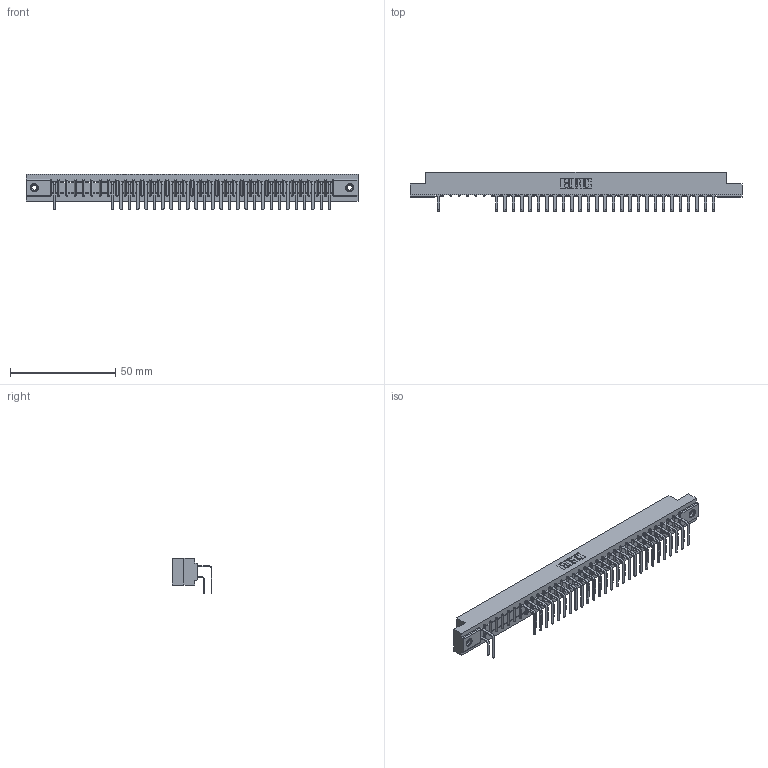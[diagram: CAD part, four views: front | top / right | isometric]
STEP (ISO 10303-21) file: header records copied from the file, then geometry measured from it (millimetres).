
FILE_DESCRIPTION (( 'STEP AP203' ), '1' );
FILE_NAME ('307-034-558-108.STEP', '2018-08-05T00:49:14', ( '' ), ( '' ), 'SwSTEP 2.0', 'SolidWorks 2016', '' );
FILE_SCHEMA (( 'CONFIG_CONTROL_DESIGN' ));
Length unit declared in the file: inch
Products named in the file (5): 307-034-558-108; 307 Part_.156 Dia Mounting Holes; 307-290-001_558 559 - 1 (Single); 307-290-001_558 - 2 (Single); 345-250-001_345-250-003-102
Assembly tree (58 placements, depth 2):
  307-034-558-108
    307 Part_.156 Dia Mounting Holes
    307-290-001_558 559 - 1 (Single)  x27
    307-290-001_558 - 2 (Single)  x28
    345-250-001_345-250-003-102  x2
Bounding box: 157.73 x 18.96 x 16.8 mm (x, y, z)
Volume: 16787.1 mm3; surface area: 20725.1 mm2
Topology: 58 solids, 58 shells, 3093 faces, 8685 edges, 5614 vertices
Faces by surface type: plane 1995, cylinder 1012, sphere 70, cone 12, torus 4
Entity records: 33438 total; most frequent: CARTESIAN_POINT 5514, ORIENTED_EDGE 5470, DIRECTION 5399, EDGE_CURVE 2735, VECTOR 2093, LINE 2093, VERTEX_POINT 1768, AXIS2_PLACEMENT_3D 1653
